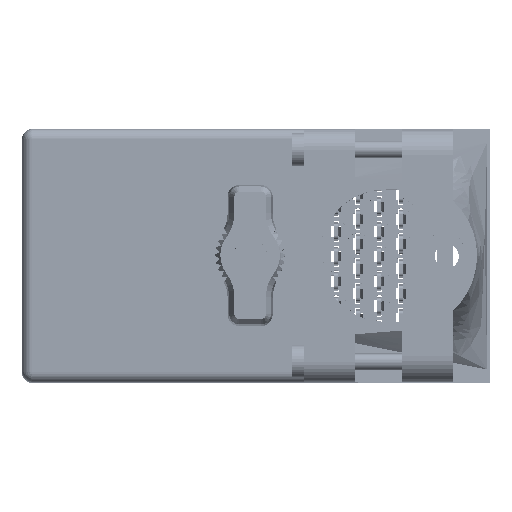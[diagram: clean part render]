
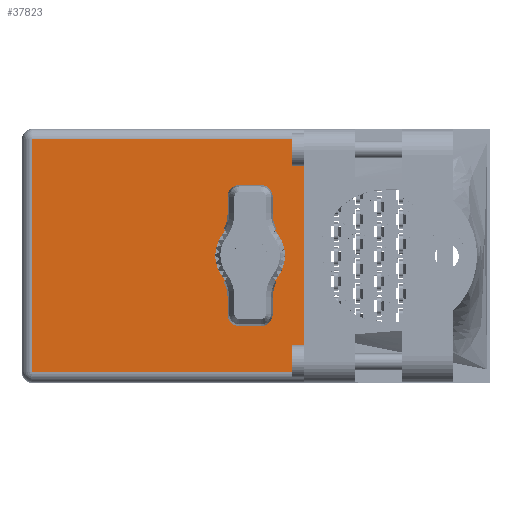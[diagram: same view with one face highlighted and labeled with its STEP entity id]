
A CAD part, top view. The second image highlights one B-rep face of the part: STEP entity #37823.
In plain terms, the highlighted face is planar.
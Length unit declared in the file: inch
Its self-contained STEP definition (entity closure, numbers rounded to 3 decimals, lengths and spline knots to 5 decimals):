
#2017 = DIRECTION ( 'NONE',  ( 0., 0., 1. ) ) ;
#3605 = CARTESIAN_POINT ( 'NONE',  ( 0.062, 2.03, -1.468 ) ) ;
#7569 = PLANE ( 'NONE',  #21551 ) ;
#10170 = CIRCLE ( 'NONE', #77323, 0.1015 ) ;
#10173 = FACE_BOUND ( 'NONE', #56896, .T. ) ;
#12189 = DIRECTION ( 'NONE',  ( 0., 0., 1. ) ) ;
#13158 = ORIENTED_EDGE ( 'NONE', *, *, #73770, .T. ) ;
#14155 = VERTEX_POINT ( 'NONE', #100376 ) ;
#14488 = CIRCLE ( 'NONE', #77509, 0.1015 ) ;
#17095 = CARTESIAN_POINT ( 'NONE',  ( 0., 2.03, -1.468 ) ) ;
#18637 = VECTOR ( 'NONE', #12189, 39.37008 ) ;
#19291 = CARTESIAN_POINT ( 'NONE',  ( 1.3775, 2.03, -0.8665 ) ) ;
#21551 = AXIS2_PLACEMENT_3D ( 'NONE', #23536, #32366, #57541 ) ;
#23536 = CARTESIAN_POINT ( 'NONE',  ( 0., 2.03, -1.53 ) ) ;
#24324 = VERTEX_POINT ( 'NONE', #19291 ) ;
#27021 = LINE ( 'NONE', #17095, #68128 ) ;
#28523 = LINE ( 'NONE', #97136, #32451 ) ;
#32269 = DIRECTION ( 'NONE',  ( 0., 0., 1. ) ) ;
#32366 = DIRECTION ( 'NONE',  ( 0., 1., 0. ) ) ;
#32451 = VECTOR ( 'NONE', #37137, 39.37008 ) ;
#37137 = DIRECTION ( 'NONE',  ( 0., 0., 1. ) ) ;
#37823 = ADVANCED_FACE ( 'NONE', ( #59216, #10173 ), #7569, .T. ) ;
#39849 = EDGE_LOOP ( 'NONE', ( #109622, #47169, #84394, #13158 ) ) ;
#41730 = ORIENTED_EDGE ( 'NONE', *, *, #105382, .F. ) ;
#43017 = ORIENTED_EDGE ( 'NONE', *, *, #49595, .F. ) ;
#46081 = EDGE_CURVE ( 'NONE', #54326, #14155, #28523, .T. ) ;
#46418 = VECTOR ( 'NONE', #95286, 39.37008 ) ;
#47169 = ORIENTED_EDGE ( 'NONE', *, *, #86554, .T. ) ;
#49595 = EDGE_CURVE ( 'NONE', #24324, #76177, #10170, .T. ) ;
#51620 = CARTESIAN_POINT ( 'NONE',  ( 1.705, 2.03, -0.062 ) ) ;
#53993 = CARTESIAN_POINT ( 'NONE',  ( 1.705, 2.03, -1.53 ) ) ;
#54326 = VERTEX_POINT ( 'NONE', #3605 ) ;
#56563 = CARTESIAN_POINT ( 'NONE',  ( 1.3775, 2.03, -0.6635 ) ) ;
#56896 = EDGE_LOOP ( 'NONE', ( #41730, #43017 ) ) ;
#56985 = LINE ( 'NONE', #53993, #18637 ) ;
#57541 = DIRECTION ( 'NONE',  ( 0., 0., 1. ) ) ;
#58200 = EDGE_CURVE ( 'NONE', #77517, #94631, #56985, .T. ) ;
#59216 = FACE_OUTER_BOUND ( 'NONE', #39849, .T. ) ;
#61914 = CARTESIAN_POINT ( 'NONE',  ( 1.3775, 2.03, -0.765 ) ) ;
#64902 = CARTESIAN_POINT ( 'NONE',  ( 1.3775, 2.03, -0.765 ) ) ;
#68128 = VECTOR ( 'NONE', #74773, 39.37008 ) ;
#68609 = CARTESIAN_POINT ( 'NONE',  ( 1.705, 2.03, -0.062 ) ) ;
#68961 = LINE ( 'NONE', #68609, #46418 ) ;
#73770 = EDGE_CURVE ( 'NONE', #77517, #54326, #27021, .T. ) ;
#74773 = DIRECTION ( 'NONE',  ( -1., 0., 0. ) ) ;
#76177 = VERTEX_POINT ( 'NONE', #56563 ) ;
#77323 = AXIS2_PLACEMENT_3D ( 'NONE', #64902, #91122, #32269 ) ;
#77509 = AXIS2_PLACEMENT_3D ( 'NONE', #61914, #78582, #2017 ) ;
#77517 = VERTEX_POINT ( 'NONE', #81057 ) ;
#78582 = DIRECTION ( 'NONE',  ( 0., 1., 0. ) ) ;
#81057 = CARTESIAN_POINT ( 'NONE',  ( 1.705, 2.03, -1.468 ) ) ;
#84394 = ORIENTED_EDGE ( 'NONE', *, *, #58200, .F. ) ;
#86554 = EDGE_CURVE ( 'NONE', #14155, #94631, #68961, .T. ) ;
#91122 = DIRECTION ( 'NONE',  ( 0., 1., 0. ) ) ;
#94631 = VERTEX_POINT ( 'NONE', #51620 ) ;
#95286 = DIRECTION ( 'NONE',  ( 1., 0., 0. ) ) ;
#97136 = CARTESIAN_POINT ( 'NONE',  ( 0.062, 2.03, -1.53 ) ) ;
#100376 = CARTESIAN_POINT ( 'NONE',  ( 0.062, 2.03, -0.062 ) ) ;
#105382 = EDGE_CURVE ( 'NONE', #76177, #24324, #14488, .T. ) ;
#109622 = ORIENTED_EDGE ( 'NONE', *, *, #46081, .T. ) ;
